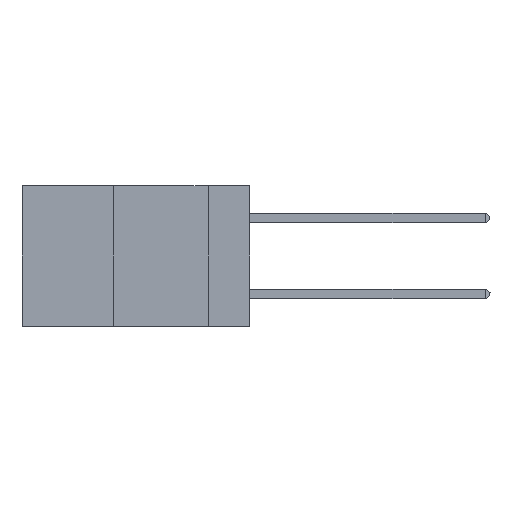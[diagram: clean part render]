
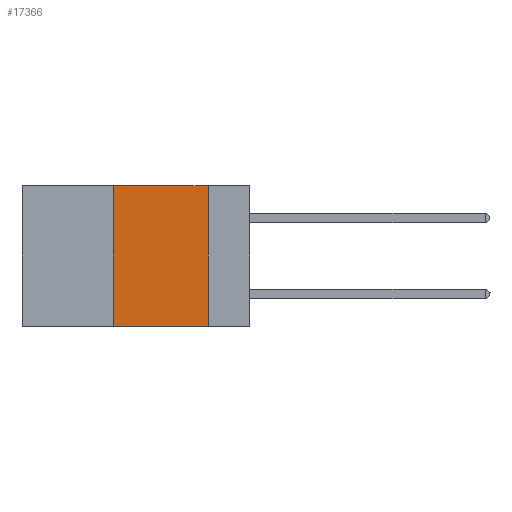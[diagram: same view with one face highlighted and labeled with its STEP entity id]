
A CAD part, left-side view. The second image highlights one B-rep face of the part: STEP entity #17366.
In plain terms, the highlighted planar face has unit normal (-1, 0, 0).
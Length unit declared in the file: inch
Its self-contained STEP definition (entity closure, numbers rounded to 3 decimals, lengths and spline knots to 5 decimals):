
#551 = FACE_OUTER_BOUND ( 'NONE', #14890, .T. ) ;
#560 = VECTOR ( 'NONE', #6982, 39.37008 ) ;
#1174 = ORIENTED_EDGE ( 'NONE', *, *, #24549, .F. ) ;
#1399 = CARTESIAN_POINT ( 'NONE',  ( 0., 0.36, -0.37 ) ) ;
#2365 = CARTESIAN_POINT ( 'NONE',  ( 0., 0.6, -0.37 ) ) ;
#2553 = CARTESIAN_POINT ( 'NONE',  ( 0., 0.11, 0. ) ) ;
#3103 = VECTOR ( 'NONE', #26969, 39.37008 ) ;
#5514 = DIRECTION ( 'NONE',  ( 0., 0., -1. ) ) ;
#6982 = DIRECTION ( 'NONE',  ( 0., 0., 1. ) ) ;
#8604 = VERTEX_POINT ( 'NONE', #27221 ) ;
#8970 = ORIENTED_EDGE ( 'NONE', *, *, #21722, .T. ) ;
#9212 = LINE ( 'NONE', #18951, #560 ) ;
#9221 = LINE ( 'NONE', #2365, #17183 ) ;
#9248 = VECTOR ( 'NONE', #15114, 39.37008 ) ;
#9654 = VERTEX_POINT ( 'NONE', #1399 ) ;
#10096 = ORIENTED_EDGE ( 'NONE', *, *, #11801, .F. ) ;
#10151 = LINE ( 'NONE', #24086, #3103 ) ;
#10606 = CARTESIAN_POINT ( 'NONE',  ( 0., 0.6, 0. ) ) ;
#11801 = EDGE_CURVE ( 'NONE', #29527, #21333, #22952, .T. ) ;
#12030 = ORIENTED_EDGE ( 'NONE', *, *, #13044, .F. ) ;
#12493 = AXIS2_PLACEMENT_3D ( 'NONE', #10606, #17799, #5514 ) ;
#13044 = EDGE_CURVE ( 'NONE', #21333, #8604, #10151, .T. ) ;
#14890 = EDGE_LOOP ( 'NONE', ( #12030, #10096, #1174, #8970 ) ) ;
#15114 = DIRECTION ( 'NONE',  ( 0., -1., 0. ) ) ;
#17183 = VECTOR ( 'NONE', #18965, 39.37008 ) ;
#17366 = ADVANCED_FACE ( 'NONE', ( #551 ), #25007, .F. ) ;
#17799 = DIRECTION ( 'NONE',  ( 1., 0., 0. ) ) ;
#17815 = CARTESIAN_POINT ( 'NONE',  ( 0., 0.6, 0. ) ) ;
#18951 = CARTESIAN_POINT ( 'NONE',  ( 0., 0.36, 0. ) ) ;
#18965 = DIRECTION ( 'NONE',  ( 0., -1., 0. ) ) ;
#21333 = VERTEX_POINT ( 'NONE', #2553 ) ;
#21722 = EDGE_CURVE ( 'NONE', #9654, #8604, #9221, .T. ) ;
#22952 = LINE ( 'NONE', #17815, #9248 ) ;
#24086 = CARTESIAN_POINT ( 'NONE',  ( 0., 0.11, 0. ) ) ;
#24549 = EDGE_CURVE ( 'NONE', #9654, #29527, #9212, .T. ) ;
#25007 = PLANE ( 'NONE',  #12493 ) ;
#25515 = CARTESIAN_POINT ( 'NONE',  ( 0., 0.36, 0. ) ) ;
#26969 = DIRECTION ( 'NONE',  ( 0., 0., -1. ) ) ;
#27221 = CARTESIAN_POINT ( 'NONE',  ( 0., 0.11, -0.37 ) ) ;
#29527 = VERTEX_POINT ( 'NONE', #25515 ) ;
